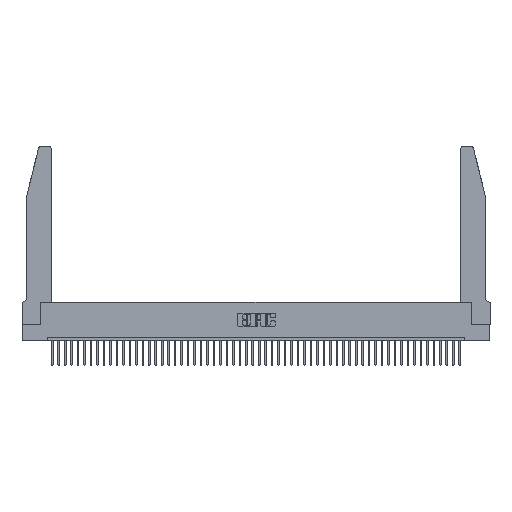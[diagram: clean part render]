
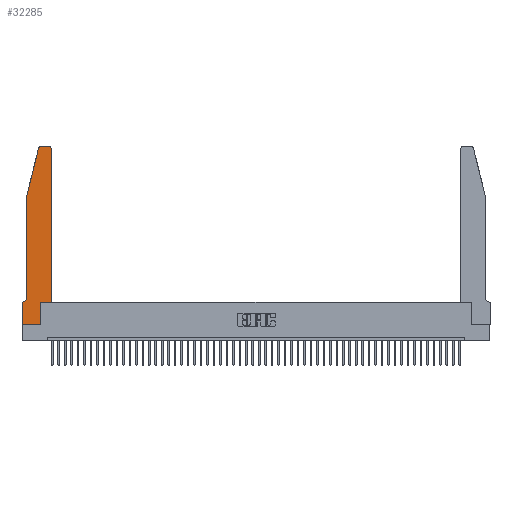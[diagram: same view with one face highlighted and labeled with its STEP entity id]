
A CAD part, top view. The second image highlights one B-rep face of the part: STEP entity #32285.
In plain terms, the highlighted planar face has unit normal (0, 0, 1).
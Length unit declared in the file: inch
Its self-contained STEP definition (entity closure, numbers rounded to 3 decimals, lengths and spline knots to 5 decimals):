
#90 = VERTEX_POINT ( 'NONE', #48729 ) ;
#171 = ORIENTED_EDGE ( 'NONE', *, *, #40763, .T. ) ;
#644 = ORIENTED_EDGE ( 'NONE', *, *, #8201, .T. ) ;
#1230 = EDGE_CURVE ( 'NONE', #39119, #43884, #1565, .T. ) ;
#1565 = CIRCLE ( 'NONE', #36482, 0.07 ) ;
#1837 = CARTESIAN_POINT ( 'NONE',  ( 0., 0., 0.37 ) ) ;
#2225 = PLANE ( 'NONE',  #42896 ) ;
#2261 = LINE ( 'NONE', #5712, #38537 ) ;
#2731 = VERTEX_POINT ( 'NONE', #16065 ) ;
#2854 = ORIENTED_EDGE ( 'NONE', *, *, #14431, .T. ) ;
#3090 = CARTESIAN_POINT ( 'NONE',  ( 0.4505, 2.72, 0.37 ) ) ;
#3230 = DIRECTION ( 'NONE',  ( -0.239, -0.971, 0. ) ) ;
#3400 = CARTESIAN_POINT ( 'NONE',  ( 0.284, 2.75, 0.37 ) ) ;
#4855 = EDGE_CURVE ( 'NONE', #30510, #8065, #42510, .T. ) ;
#5304 = VECTOR ( 'NONE', #47559, 39.37008 ) ;
#5327 = ORIENTED_EDGE ( 'NONE', *, *, #4855, .T. ) ;
#5712 = CARTESIAN_POINT ( 'NONE',  ( 0.4505, 0.35, 0.37 ) ) ;
#7553 = VECTOR ( 'NONE', #23040, 39.37008 ) ;
#7868 = CARTESIAN_POINT ( 'NONE',  ( 0.0755, 0.35, 0.37 ) ) ;
#8065 = VERTEX_POINT ( 'NONE', #3090 ) ;
#8201 = EDGE_CURVE ( 'NONE', #2731, #20482, #49815, .T. ) ;
#8355 = CARTESIAN_POINT ( 'NONE',  ( 0.4505, 0.35, 0.37 ) ) ;
#11267 = CARTESIAN_POINT ( 'NONE',  ( 0., 0., 0.37 ) ) ;
#11701 = CIRCLE ( 'NONE', #37981, 0.03 ) ;
#12018 = CARTESIAN_POINT ( 'NONE',  ( 0., 0., 0.37 ) ) ;
#12050 = CARTESIAN_POINT ( 'NONE',  ( 0.4205, 2.72, 0.37 ) ) ;
#12060 = EDGE_CURVE ( 'NONE', #18894, #30510, #2261, .T. ) ;
#13761 = CARTESIAN_POINT ( 'NONE',  ( 0., 0.35, 0.37 ) ) ;
#14431 = EDGE_CURVE ( 'NONE', #20482, #90, #23907, .T. ) ;
#14915 = DIRECTION ( 'NONE',  ( 1., 0., 0. ) ) ;
#15368 = ORIENTED_EDGE ( 'NONE', *, *, #44922, .T. ) ;
#16065 = CARTESIAN_POINT ( 'NONE',  ( 0., 0.35, 0.37 ) ) ;
#16242 = CARTESIAN_POINT ( 'NONE',  ( 0.4205, 2.75, 0.37 ) ) ;
#16807 = LINE ( 'NONE', #7868, #5304 ) ;
#17241 = CARTESIAN_POINT ( 'NONE',  ( 0.2605, 2.75, 0.37 ) ) ;
#17391 = CARTESIAN_POINT ( 'NONE',  ( 0.0755, 0.42, 0.37 ) ) ;
#17490 = CARTESIAN_POINT ( 'NONE',  ( 0.2865, 0.35, 0.37 ) ) ;
#17518 = ORIENTED_EDGE ( 'NONE', *, *, #1230, .T. ) ;
#17787 = CARTESIAN_POINT ( 'NONE',  ( 0.284, 2.72, 0.37 ) ) ;
#18208 = CARTESIAN_POINT ( 'NONE',  ( 0.25487, 2.72718, 0.37 ) ) ;
#18894 = VERTEX_POINT ( 'NONE', #21465 ) ;
#18987 = CARTESIAN_POINT ( 'NONE',  ( 0.0755, 2., 0.37 ) ) ;
#19474 = DIRECTION ( 'NONE',  ( 0., 1., 0. ) ) ;
#20482 = VERTEX_POINT ( 'NONE', #1837 ) ;
#21101 = LINE ( 'NONE', #17490, #44047 ) ;
#21465 = CARTESIAN_POINT ( 'NONE',  ( 0.2865, 0.35, 0.37 ) ) ;
#21782 = EDGE_CURVE ( 'NONE', #21810, #39119, #27161, .T. ) ;
#21810 = VERTEX_POINT ( 'NONE', #27807 ) ;
#23040 = DIRECTION ( 'NONE',  ( 0., 1., 0. ) ) ;
#23626 = DIRECTION ( 'NONE',  ( -1., 0., 0. ) ) ;
#23907 = LINE ( 'NONE', #12018, #42073 ) ;
#24890 = ORIENTED_EDGE ( 'NONE', *, *, #28248, .T. ) ;
#24941 = VECTOR ( 'NONE', #3230, 39.37008 ) ;
#25958 = VECTOR ( 'NONE', #49636, 39.37008 ) ;
#26004 = CARTESIAN_POINT ( 'NONE',  ( 0.0755, 2., 0.37 ) ) ;
#26201 = LINE ( 'NONE', #26004, #24941 ) ;
#26339 = EDGE_LOOP ( 'NONE', ( #47863, #24890, #39739, #40496, #17518, #47471, #644, #2854, #15368, #46293, #5327, #171 ) ) ;
#26907 = VERTEX_POINT ( 'NONE', #18208 ) ;
#27161 = LINE ( 'NONE', #18987, #25958 ) ;
#27807 = CARTESIAN_POINT ( 'NONE',  ( 0.0755, 2., 0.37 ) ) ;
#27966 = EDGE_CURVE ( 'NONE', #26907, #21810, #26201, .T. ) ;
#28248 = EDGE_CURVE ( 'NONE', #47173, #26907, #11701, .T. ) ;
#30510 = VERTEX_POINT ( 'NONE', #8355 ) ;
#30774 = VECTOR ( 'NONE', #40140, 39.37008 ) ;
#31082 = DIRECTION ( 'NONE',  ( 0., 0., -1. ) ) ;
#31160 = CIRCLE ( 'NONE', #33863, 0.03 ) ;
#32285 = ADVANCED_FACE ( 'NONE', ( #42615 ), #2225, .T. ) ;
#33863 = AXIS2_PLACEMENT_3D ( 'NONE', #12050, #39339, #47066 ) ;
#36482 = AXIS2_PLACEMENT_3D ( 'NONE', #46741, #31082, #23626 ) ;
#36984 = CARTESIAN_POINT ( 'NONE',  ( 0.0055, 0.35, 0.37 ) ) ;
#37787 = EDGE_CURVE ( 'NONE', #43884, #2731, #16807, .T. ) ;
#37981 = AXIS2_PLACEMENT_3D ( 'NONE', #17787, #44742, #14915 ) ;
#38246 = DIRECTION ( 'NONE',  ( 0., -1., 0. ) ) ;
#38537 = VECTOR ( 'NONE', #40790, 39.37008 ) ;
#39119 = VERTEX_POINT ( 'NONE', #17391 ) ;
#39339 = DIRECTION ( 'NONE',  ( 0., 0., 1. ) ) ;
#39739 = ORIENTED_EDGE ( 'NONE', *, *, #27966, .T. ) ;
#40140 = DIRECTION ( 'NONE',  ( -1., 0., 0. ) ) ;
#40496 = ORIENTED_EDGE ( 'NONE', *, *, #21782, .T. ) ;
#40719 = DIRECTION ( 'NONE',  ( 0., 0., 1. ) ) ;
#40763 = EDGE_CURVE ( 'NONE', #8065, #44716, #31160, .T. ) ;
#40790 = DIRECTION ( 'NONE',  ( 1., 0., 0. ) ) ;
#41032 = LINE ( 'NONE', #17241, #30774 ) ;
#42073 = VECTOR ( 'NONE', #42855, 39.37008 ) ;
#42510 = LINE ( 'NONE', #42603, #7553 ) ;
#42603 = CARTESIAN_POINT ( 'NONE',  ( 0.4505, 0.35, 0.37 ) ) ;
#42615 = FACE_OUTER_BOUND ( 'NONE', #26339, .T. ) ;
#42855 = DIRECTION ( 'NONE',  ( 1., 0., 0. ) ) ;
#42896 = AXIS2_PLACEMENT_3D ( 'NONE', #13761, #40719, #44941 ) ;
#43884 = VERTEX_POINT ( 'NONE', #36984 ) ;
#44047 = VECTOR ( 'NONE', #19474, 39.37008 ) ;
#44716 = VERTEX_POINT ( 'NONE', #16242 ) ;
#44742 = DIRECTION ( 'NONE',  ( 0., 0., 1. ) ) ;
#44922 = EDGE_CURVE ( 'NONE', #90, #18894, #21101, .T. ) ;
#44941 = DIRECTION ( 'NONE',  ( 1., 0., 0. ) ) ;
#46181 = EDGE_CURVE ( 'NONE', #44716, #47173, #41032, .T. ) ;
#46293 = ORIENTED_EDGE ( 'NONE', *, *, #12060, .T. ) ;
#46723 = VECTOR ( 'NONE', #38246, 39.37008 ) ;
#46741 = CARTESIAN_POINT ( 'NONE',  ( 0.0055, 0.42, 0.37 ) ) ;
#47066 = DIRECTION ( 'NONE',  ( 1., 0., 0. ) ) ;
#47173 = VERTEX_POINT ( 'NONE', #3400 ) ;
#47471 = ORIENTED_EDGE ( 'NONE', *, *, #37787, .T. ) ;
#47559 = DIRECTION ( 'NONE',  ( -1., 0., 0. ) ) ;
#47863 = ORIENTED_EDGE ( 'NONE', *, *, #46181, .T. ) ;
#48729 = CARTESIAN_POINT ( 'NONE',  ( 0.2865, 0., 0.37 ) ) ;
#49636 = DIRECTION ( 'NONE',  ( 0., -1., 0. ) ) ;
#49815 = LINE ( 'NONE', #11267, #46723 ) ;
